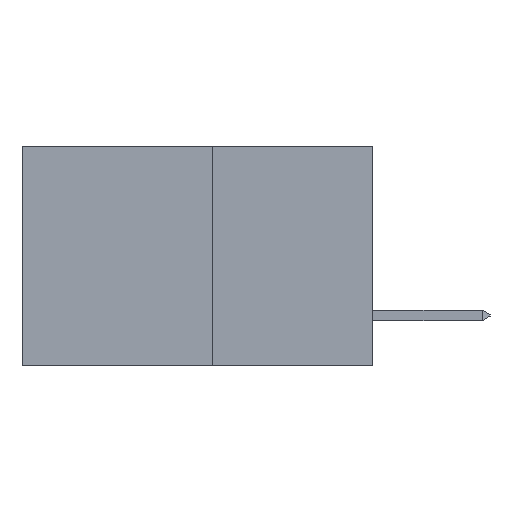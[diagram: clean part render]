
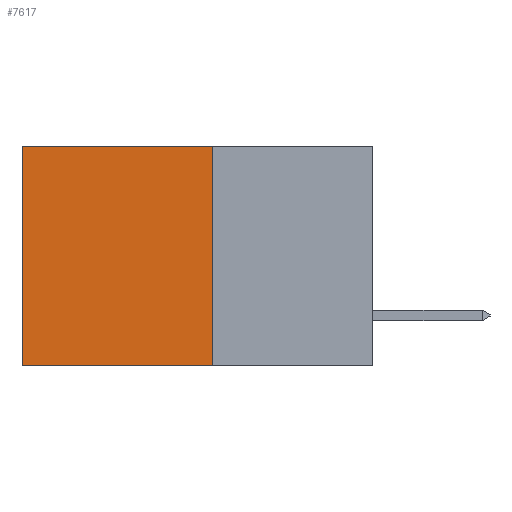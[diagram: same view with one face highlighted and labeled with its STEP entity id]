
A CAD part, left-side view. The second image highlights one B-rep face of the part: STEP entity #7617.
In plain terms, the highlighted planar face has unit normal (-1, 0, 0).
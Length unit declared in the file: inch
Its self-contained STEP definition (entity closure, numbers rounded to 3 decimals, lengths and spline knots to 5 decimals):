
#74 = VERTEX_POINT ( 'NONE', #9816 ) ;
#105 = DIRECTION ( 'NONE',  ( 0., 0., -1. ) ) ;
#160 = EDGE_CURVE ( 'NONE', #3289, #74, #643, .T. ) ;
#589 = EDGE_CURVE ( 'NONE', #74, #8608, #5574, .T. ) ;
#643 = LINE ( 'NONE', #5506, #7479 ) ;
#718 = ORIENTED_EDGE ( 'NONE', *, *, #160, .T. ) ;
#886 = VECTOR ( 'NONE', #8619, 39.37008 ) ;
#982 = DIRECTION ( 'NONE',  ( 0., 0., -1. ) ) ;
#1115 = CARTESIAN_POINT ( 'NONE',  ( 0.277, 0.27, -0.37 ) ) ;
#1276 = CARTESIAN_POINT ( 'NONE',  ( 0.277, 0.59, -0.37 ) ) ;
#1351 = AXIS2_PLACEMENT_3D ( 'NONE', #3543, #5130, #105 ) ;
#1459 = DIRECTION ( 'NONE',  ( 0., 0., -1. ) ) ;
#2184 = CARTESIAN_POINT ( 'NONE',  ( 0.277, 0.27, -0.37 ) ) ;
#2757 = ORIENTED_EDGE ( 'NONE', *, *, #5529, .F. ) ;
#2914 = LINE ( 'NONE', #2184, #886 ) ;
#3289 = VERTEX_POINT ( 'NONE', #4764 ) ;
#3539 = EDGE_LOOP ( 'NONE', ( #4425, #8908, #2757, #718 ) ) ;
#3543 = CARTESIAN_POINT ( 'NONE',  ( 0.277, 0.27, -0.37 ) ) ;
#3954 = VERTEX_POINT ( 'NONE', #8937 ) ;
#3999 = CARTESIAN_POINT ( 'NONE',  ( 0.277, 0.59, -0.37 ) ) ;
#4337 = PLANE ( 'NONE',  #1351 ) ;
#4425 = ORIENTED_EDGE ( 'NONE', *, *, #589, .T. ) ;
#4764 = CARTESIAN_POINT ( 'NONE',  ( 0.277, 0.27, 0. ) ) ;
#5130 = DIRECTION ( 'NONE',  ( 1., 0., 0. ) ) ;
#5498 = DIRECTION ( 'NONE',  ( 0., 1., 0. ) ) ;
#5506 = CARTESIAN_POINT ( 'NONE',  ( 0.277, 0.27, 0. ) ) ;
#5529 = EDGE_CURVE ( 'NONE', #3289, #3954, #7986, .T. ) ;
#5574 = LINE ( 'NONE', #1276, #7470 ) ;
#7470 = VECTOR ( 'NONE', #1459, 39.37008 ) ;
#7479 = VECTOR ( 'NONE', #5498, 39.37008 ) ;
#7617 = ADVANCED_FACE ( 'NONE', ( #9094 ), #4337, .F. ) ;
#7986 = LINE ( 'NONE', #1115, #9788 ) ;
#8608 = VERTEX_POINT ( 'NONE', #3999 ) ;
#8619 = DIRECTION ( 'NONE',  ( 0., 1., 0. ) ) ;
#8908 = ORIENTED_EDGE ( 'NONE', *, *, #10335, .F. ) ;
#8937 = CARTESIAN_POINT ( 'NONE',  ( 0.277, 0.27, -0.37 ) ) ;
#9094 = FACE_OUTER_BOUND ( 'NONE', #3539, .T. ) ;
#9788 = VECTOR ( 'NONE', #982, 39.37008 ) ;
#9816 = CARTESIAN_POINT ( 'NONE',  ( 0.277, 0.59, 0. ) ) ;
#10335 = EDGE_CURVE ( 'NONE', #3954, #8608, #2914, .T. ) ;
